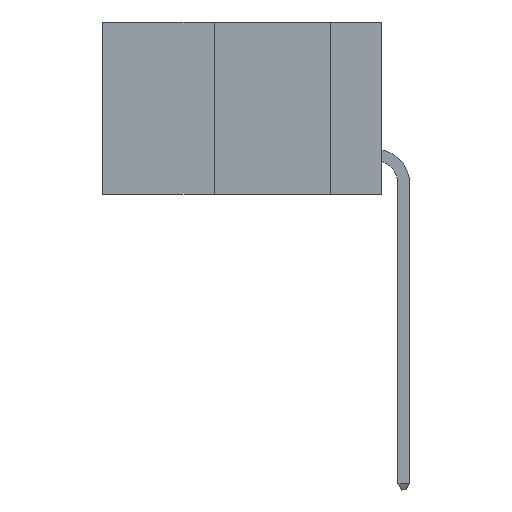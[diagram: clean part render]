
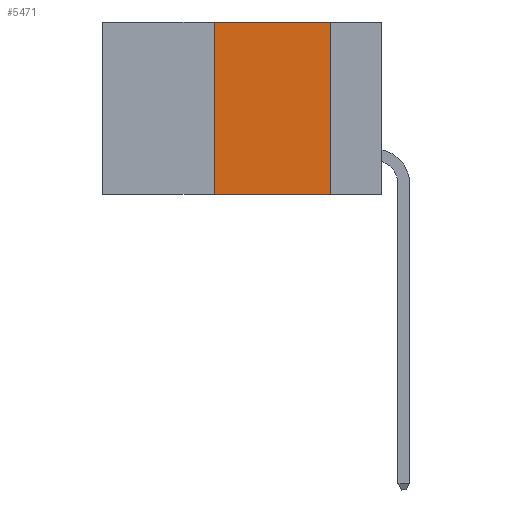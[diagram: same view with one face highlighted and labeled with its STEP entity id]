
A CAD part, left-side view. The second image highlights one B-rep face of the part: STEP entity #5471.
In plain terms, the highlighted planar face has unit normal (-1, 0, 0).
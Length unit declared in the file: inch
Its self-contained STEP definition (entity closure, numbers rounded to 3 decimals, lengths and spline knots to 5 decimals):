
#75 = CARTESIAN_POINT ( 'NONE',  ( 0., 0.36, -0.37 ) ) ;
#105 = CARTESIAN_POINT ( 'NONE',  ( 0., 0.6, 0. ) ) ;
#160 = PLANE ( 'NONE',  #50129 ) ;
#2567 = ORIENTED_EDGE ( 'NONE', *, *, #21423, .T. ) ;
#2608 = VERTEX_POINT ( 'NONE', #75 ) ;
#3374 = LINE ( 'NONE', #46678, #34997 ) ;
#4169 = DIRECTION ( 'NONE',  ( 0., 0., -1. ) ) ;
#5471 = ADVANCED_FACE ( 'NONE', ( #24895 ), #160, .F. ) ;
#6000 = DIRECTION ( 'NONE',  ( 0., 0., 1. ) ) ;
#6726 = DIRECTION ( 'NONE',  ( 1., 0., 0. ) ) ;
#6995 = LINE ( 'NONE', #49296, #16021 ) ;
#7464 = VECTOR ( 'NONE', #6000, 39.37008 ) ;
#8585 = ORIENTED_EDGE ( 'NONE', *, *, #19734, .F. ) ;
#11377 = VERTEX_POINT ( 'NONE', #26169 ) ;
#13467 = LINE ( 'NONE', #21425, #7464 ) ;
#15007 = EDGE_CURVE ( 'NONE', #27721, #11377, #3374, .T. ) ;
#15136 = CARTESIAN_POINT ( 'NONE',  ( 0., 0.36, 0. ) ) ;
#16021 = VECTOR ( 'NONE', #27041, 39.37008 ) ;
#16391 = VECTOR ( 'NONE', #18048, 39.37008 ) ;
#18042 = ORIENTED_EDGE ( 'NONE', *, *, #15007, .F. ) ;
#18048 = DIRECTION ( 'NONE',  ( 0., -1., 0. ) ) ;
#19734 = EDGE_CURVE ( 'NONE', #2608, #38025, #13467, .T. ) ;
#21423 = EDGE_CURVE ( 'NONE', #2608, #11377, #31083, .T. ) ;
#21425 = CARTESIAN_POINT ( 'NONE',  ( 0., 0.36, 0. ) ) ;
#24895 = FACE_OUTER_BOUND ( 'NONE', #33659, .T. ) ;
#26169 = CARTESIAN_POINT ( 'NONE',  ( 0., 0.11, -0.37 ) ) ;
#27041 = DIRECTION ( 'NONE',  ( 0., -1., 0. ) ) ;
#27123 = CARTESIAN_POINT ( 'NONE',  ( 0., 0.6, -0.37 ) ) ;
#27721 = VERTEX_POINT ( 'NONE', #43002 ) ;
#31083 = LINE ( 'NONE', #27123, #16391 ) ;
#33659 = EDGE_LOOP ( 'NONE', ( #18042, #44809, #8585, #2567 ) ) ;
#34997 = VECTOR ( 'NONE', #4169, 39.37008 ) ;
#38025 = VERTEX_POINT ( 'NONE', #15136 ) ;
#39538 = EDGE_CURVE ( 'NONE', #38025, #27721, #6995, .T. ) ;
#39651 = DIRECTION ( 'NONE',  ( 0., 0., -1. ) ) ;
#43002 = CARTESIAN_POINT ( 'NONE',  ( 0., 0.11, 0. ) ) ;
#44809 = ORIENTED_EDGE ( 'NONE', *, *, #39538, .F. ) ;
#46678 = CARTESIAN_POINT ( 'NONE',  ( 0., 0.11, 0. ) ) ;
#49296 = CARTESIAN_POINT ( 'NONE',  ( 0., 0.6, 0. ) ) ;
#50129 = AXIS2_PLACEMENT_3D ( 'NONE', #105, #6726, #39651 ) ;
